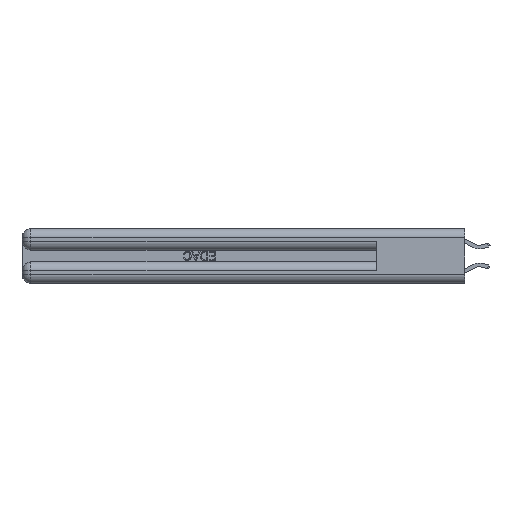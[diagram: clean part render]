
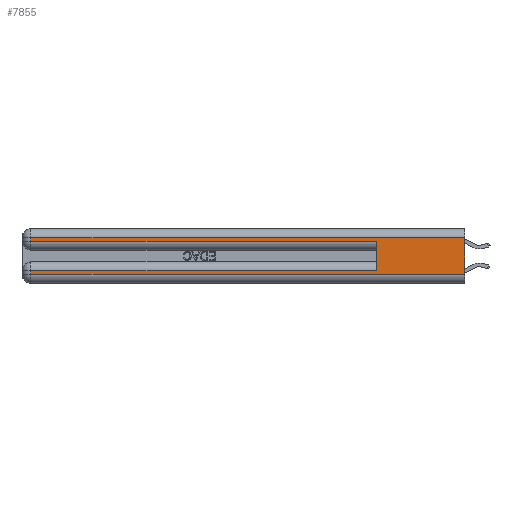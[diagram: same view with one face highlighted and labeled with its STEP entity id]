
A CAD part, left-side view. The second image highlights one B-rep face of the part: STEP entity #7855.
In plain terms, the highlighted planar face has unit normal (-1, 0, 0).
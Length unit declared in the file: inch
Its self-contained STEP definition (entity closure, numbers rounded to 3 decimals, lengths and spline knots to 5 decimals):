
#375 = DIRECTION ( 'NONE',  ( 0., 0., -1. ) ) ;
#445 = VECTOR ( 'NONE', #21224, 39.37008 ) ;
#912 = EDGE_CURVE ( 'NONE', #29149, #15085, #5302, .T. ) ;
#1163 = CARTESIAN_POINT ( 'NONE',  ( 0., 0., 0.285 ) ) ;
#2289 = VERTEX_POINT ( 'NONE', #27796 ) ;
#3737 = ORIENTED_EDGE ( 'NONE', *, *, #20863, .F. ) ;
#4125 = DIRECTION ( 'NONE',  ( 0., 1., 0. ) ) ;
#4358 = VECTOR ( 'NONE', #20353, 39.37008 ) ;
#4899 = CARTESIAN_POINT ( 'NONE',  ( 0., 0., 0.37 ) ) ;
#4996 = DIRECTION ( 'NONE',  ( 0., 0., -1. ) ) ;
#5095 = CARTESIAN_POINT ( 'NONE',  ( 0., 0., 0.31 ) ) ;
#5273 = DIRECTION ( 'NONE',  ( 1., 0., 0. ) ) ;
#5302 = LINE ( 'NONE', #17967, #7128 ) ;
#5402 = ORIENTED_EDGE ( 'NONE', *, *, #23799, .T. ) ;
#6042 = VERTEX_POINT ( 'NONE', #14844 ) ;
#6119 = VECTOR ( 'NONE', #12730, 39.37008 ) ;
#6165 = VERTEX_POINT ( 'NONE', #8331 ) ;
#6287 = DIRECTION ( 'NONE',  ( 0., 0., -1. ) ) ;
#6670 = VERTEX_POINT ( 'NONE', #5095 ) ;
#7128 = VECTOR ( 'NONE', #6287, 39.37008 ) ;
#7253 = CARTESIAN_POINT ( 'NONE',  ( 0., 0., 0.06 ) ) ;
#7855 = ADVANCED_FACE ( 'NONE', ( #28154 ), #14304, .F. ) ;
#8331 = CARTESIAN_POINT ( 'NONE',  ( 0., 0.6, 0.285 ) ) ;
#9239 = CARTESIAN_POINT ( 'NONE',  ( 0., 0.6, 0.145 ) ) ;
#9507 = VERTEX_POINT ( 'NONE', #10776 ) ;
#9835 = ORIENTED_EDGE ( 'NONE', *, *, #14140, .T. ) ;
#9916 = EDGE_CURVE ( 'NONE', #2289, #14679, #23906, .T. ) ;
#10457 = CARTESIAN_POINT ( 'NONE',  ( 0., 0., 0.37 ) ) ;
#10592 = LINE ( 'NONE', #10457, #4358 ) ;
#10776 = CARTESIAN_POINT ( 'NONE',  ( 0., 2.94, 0.06 ) ) ;
#11290 = LINE ( 'NONE', #1163, #6119 ) ;
#12120 = VECTOR ( 'NONE', #16158, 39.37008 ) ;
#12730 = DIRECTION ( 'NONE',  ( 0., -1., 0. ) ) ;
#13066 = EDGE_CURVE ( 'NONE', #2289, #6165, #17217, .T. ) ;
#13136 = CARTESIAN_POINT ( 'NONE',  ( 0., 0., 0.31 ) ) ;
#13274 = VECTOR ( 'NONE', #375, 39.37008 ) ;
#14140 = EDGE_CURVE ( 'NONE', #15085, #6165, #11290, .T. ) ;
#14187 = ORIENTED_EDGE ( 'NONE', *, *, #13066, .F. ) ;
#14304 = PLANE ( 'NONE',  #29447 ) ;
#14679 = VERTEX_POINT ( 'NONE', #19846 ) ;
#14844 = CARTESIAN_POINT ( 'NONE',  ( 0., 0., 0.06 ) ) ;
#15085 = VERTEX_POINT ( 'NONE', #19677 ) ;
#15200 = EDGE_CURVE ( 'NONE', #6670, #29149, #15260, .T. ) ;
#15260 = LINE ( 'NONE', #13136, #25109 ) ;
#15823 = LINE ( 'NONE', #25995, #13274 ) ;
#16000 = ORIENTED_EDGE ( 'NONE', *, *, #9916, .T. ) ;
#16158 = DIRECTION ( 'NONE',  ( 0., 0., 1. ) ) ;
#16989 = VECTOR ( 'NONE', #29994, 39.37008 ) ;
#17217 = LINE ( 'NONE', #9239, #12120 ) ;
#17967 = CARTESIAN_POINT ( 'NONE',  ( 0., 2.94, 0.37 ) ) ;
#19067 = ORIENTED_EDGE ( 'NONE', *, *, #30012, .T. ) ;
#19113 = LINE ( 'NONE', #7253, #445 ) ;
#19677 = CARTESIAN_POINT ( 'NONE',  ( 0., 2.94, 0.285 ) ) ;
#19780 = ORIENTED_EDGE ( 'NONE', *, *, #15200, .T. ) ;
#19846 = CARTESIAN_POINT ( 'NONE',  ( 0., 2.94, 0.085 ) ) ;
#20353 = DIRECTION ( 'NONE',  ( 0., 0., -1. ) ) ;
#20863 = EDGE_CURVE ( 'NONE', #6670, #6042, #10592, .T. ) ;
#21224 = DIRECTION ( 'NONE',  ( 0., -1., 0. ) ) ;
#23799 = EDGE_CURVE ( 'NONE', #14679, #9507, #15823, .T. ) ;
#23906 = LINE ( 'NONE', #25289, #16989 ) ;
#25109 = VECTOR ( 'NONE', #4125, 39.37008 ) ;
#25289 = CARTESIAN_POINT ( 'NONE',  ( 0., 0., 0.085 ) ) ;
#25995 = CARTESIAN_POINT ( 'NONE',  ( 0., 2.94, 0.37 ) ) ;
#26168 = CARTESIAN_POINT ( 'NONE',  ( 0., 2.94, 0.31 ) ) ;
#26983 = ORIENTED_EDGE ( 'NONE', *, *, #912, .T. ) ;
#27796 = CARTESIAN_POINT ( 'NONE',  ( 0., 0.6, 0.085 ) ) ;
#28154 = FACE_OUTER_BOUND ( 'NONE', #30246, .T. ) ;
#29149 = VERTEX_POINT ( 'NONE', #26168 ) ;
#29447 = AXIS2_PLACEMENT_3D ( 'NONE', #4899, #5273, #4996 ) ;
#29994 = DIRECTION ( 'NONE',  ( 0., 1., 0. ) ) ;
#30012 = EDGE_CURVE ( 'NONE', #9507, #6042, #19113, .T. ) ;
#30246 = EDGE_LOOP ( 'NONE', ( #3737, #19780, #26983, #9835, #14187, #16000, #5402, #19067 ) ) ;
